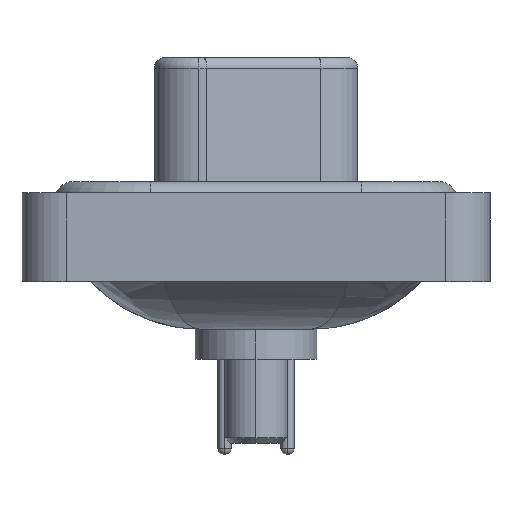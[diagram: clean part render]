
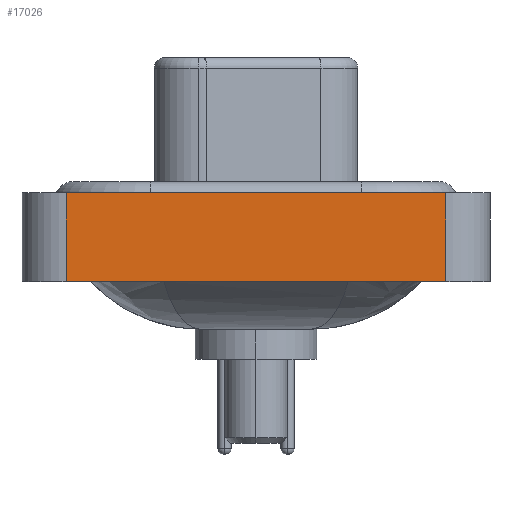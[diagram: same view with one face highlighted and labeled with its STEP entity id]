
A CAD part, left-side view. The second image highlights one B-rep face of the part: STEP entity #17026.
In plain terms, the highlighted planar face has unit normal (-1, 0, 0).
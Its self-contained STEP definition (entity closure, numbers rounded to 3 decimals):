
#851 = ORIENTED_EDGE ( 'NONE', *, *, #18334, .T. ) ;
#1777 = AXIS2_PLACEMENT_3D ( 'NONE', #9229, #10934, #14285 ) ;
#2428 = CARTESIAN_POINT ( 'NONE',  ( -7.35, -8.55, 0.4 ) ) ;
#3821 = CARTESIAN_POINT ( 'NONE',  ( -7.35, -8.55, 0.4 ) ) ;
#4735 = PLANE ( 'NONE',  #1777 ) ;
#4760 = VECTOR ( 'NONE', #15164, 1000. ) ;
#4780 = CARTESIAN_POINT ( 'NONE',  ( -7.35, 8.55, 0.4 ) ) ;
#5150 = EDGE_CURVE ( 'NONE', #7631, #11224, #7192, .T. ) ;
#5186 = VERTEX_POINT ( 'NONE', #7397 ) ;
#5399 = EDGE_LOOP ( 'NONE', ( #8179, #15510, #15793, #851 ) ) ;
#5577 = LINE ( 'NONE', #8450, #9814 ) ;
#5690 = CARTESIAN_POINT ( 'NONE',  ( -7.35, -8.55, -3.6 ) ) ;
#6124 = FACE_OUTER_BOUND ( 'NONE', #5399, .T. ) ;
#6898 = VECTOR ( 'NONE', #14415, 1000. ) ;
#7063 = DIRECTION ( 'NONE',  ( 0., 0., 1. ) ) ;
#7192 = LINE ( 'NONE', #5690, #16104 ) ;
#7397 = CARTESIAN_POINT ( 'NONE',  ( -7.35, 8.55, -3.6 ) ) ;
#7631 = VERTEX_POINT ( 'NONE', #14802 ) ;
#7819 = EDGE_CURVE ( 'NONE', #5186, #16706, #5577, .T. ) ;
#8179 = ORIENTED_EDGE ( 'NONE', *, *, #5150, .T. ) ;
#8450 = CARTESIAN_POINT ( 'NONE',  ( -7.35, 8.55, -3.6 ) ) ;
#9229 = CARTESIAN_POINT ( 'NONE',  ( -7.35, -8.55, -3.6 ) ) ;
#9814 = VECTOR ( 'NONE', #7063, 1000. ) ;
#10934 = DIRECTION ( 'NONE',  ( -1., 0., 0. ) ) ;
#10957 = LINE ( 'NONE', #17392, #6898 ) ;
#11224 = VERTEX_POINT ( 'NONE', #3821 ) ;
#11349 = EDGE_CURVE ( 'NONE', #16706, #11224, #12141, .T. ) ;
#12141 = LINE ( 'NONE', #2428, #4760 ) ;
#14285 = DIRECTION ( 'NONE',  ( 0., 0., 1. ) ) ;
#14415 = DIRECTION ( 'NONE',  ( 0., -1., 0. ) ) ;
#14802 = CARTESIAN_POINT ( 'NONE',  ( -7.35, -8.55, -3.6 ) ) ;
#15164 = DIRECTION ( 'NONE',  ( 0., -1., 0. ) ) ;
#15350 = DIRECTION ( 'NONE',  ( 0., 0., 1. ) ) ;
#15510 = ORIENTED_EDGE ( 'NONE', *, *, #11349, .F. ) ;
#15793 = ORIENTED_EDGE ( 'NONE', *, *, #7819, .F. ) ;
#16104 = VECTOR ( 'NONE', #15350, 1000. ) ;
#16706 = VERTEX_POINT ( 'NONE', #4780 ) ;
#17026 = ADVANCED_FACE ( 'NONE', ( #6124 ), #4735, .T. ) ;
#17392 = CARTESIAN_POINT ( 'NONE',  ( -7.35, -8.55, -3.6 ) ) ;
#18334 = EDGE_CURVE ( 'NONE', #5186, #7631, #10957, .T. ) ;
